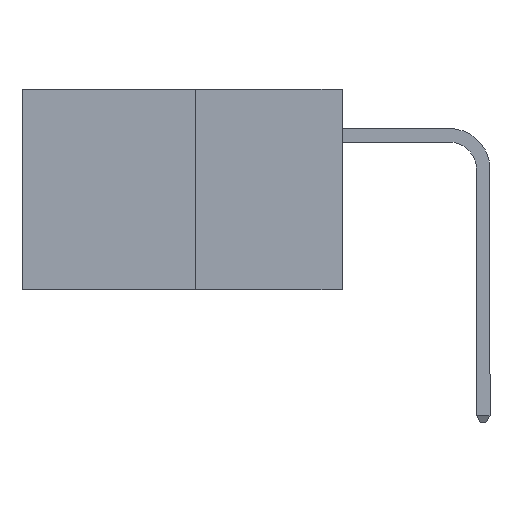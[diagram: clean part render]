
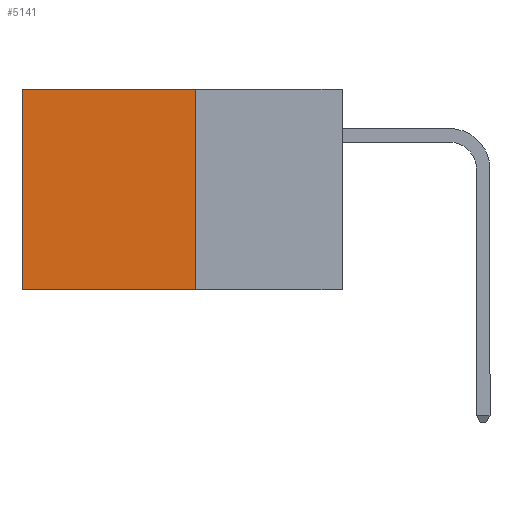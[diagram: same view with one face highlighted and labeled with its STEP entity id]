
A CAD part, left-side view. The second image highlights one B-rep face of the part: STEP entity #5141.
In plain terms, the highlighted planar face has unit normal (-1, 0, 0).
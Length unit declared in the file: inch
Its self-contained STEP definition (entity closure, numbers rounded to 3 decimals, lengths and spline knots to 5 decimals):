
#7 = LINE ( 'NONE', #8174, #3873 ) ;
#1170 = EDGE_LOOP ( 'NONE', ( #4244, #2759, #6748, #7201 ) ) ;
#1661 = VERTEX_POINT ( 'NONE', #3243 ) ;
#1672 = EDGE_CURVE ( 'NONE', #7537, #4036, #6747, .T. ) ;
#1724 = VERTEX_POINT ( 'NONE', #7793 ) ;
#2165 = LINE ( 'NONE', #4706, #3596 ) ;
#2404 = VECTOR ( 'NONE', #2428, 39.37008 ) ;
#2428 = DIRECTION ( 'NONE',  ( 0., 0., -1. ) ) ;
#2453 = EDGE_CURVE ( 'NONE', #1661, #1724, #7, .T. ) ;
#2570 = CARTESIAN_POINT ( 'NONE',  ( 0.277, 0.59, -0.37 ) ) ;
#2619 = LINE ( 'NONE', #6888, #2404 ) ;
#2759 = ORIENTED_EDGE ( 'NONE', *, *, #1672, .F. ) ;
#3243 = CARTESIAN_POINT ( 'NONE',  ( 0.277, 0.27, 0. ) ) ;
#3267 = DIRECTION ( 'NONE',  ( 0., 1., 0. ) ) ;
#3596 = VECTOR ( 'NONE', #3936, 39.37008 ) ;
#3873 = VECTOR ( 'NONE', #5328, 39.37008 ) ;
#3936 = DIRECTION ( 'NONE',  ( 0., 0., -1. ) ) ;
#4036 = VERTEX_POINT ( 'NONE', #2570 ) ;
#4162 = CARTESIAN_POINT ( 'NONE',  ( 0.277, 0.27, -0.37 ) ) ;
#4244 = ORIENTED_EDGE ( 'NONE', *, *, #9126, .T. ) ;
#4706 = CARTESIAN_POINT ( 'NONE',  ( 0.277, 0.59, -0.37 ) ) ;
#5141 = ADVANCED_FACE ( 'NONE', ( #9236 ), #7254, .F. ) ;
#5328 = DIRECTION ( 'NONE',  ( 0., 1., 0. ) ) ;
#6203 = AXIS2_PLACEMENT_3D ( 'NONE', #7246, #7221, #7155 ) ;
#6336 = CARTESIAN_POINT ( 'NONE',  ( 0.277, 0.27, -0.37 ) ) ;
#6747 = LINE ( 'NONE', #6336, #7200 ) ;
#6748 = ORIENTED_EDGE ( 'NONE', *, *, #9047, .F. ) ;
#6888 = CARTESIAN_POINT ( 'NONE',  ( 0.277, 0.27, -0.37 ) ) ;
#7155 = DIRECTION ( 'NONE',  ( 0., 0., -1. ) ) ;
#7200 = VECTOR ( 'NONE', #3267, 39.37008 ) ;
#7201 = ORIENTED_EDGE ( 'NONE', *, *, #2453, .T. ) ;
#7221 = DIRECTION ( 'NONE',  ( 1., 0., 0. ) ) ;
#7246 = CARTESIAN_POINT ( 'NONE',  ( 0.277, 0.27, -0.37 ) ) ;
#7254 = PLANE ( 'NONE',  #6203 ) ;
#7537 = VERTEX_POINT ( 'NONE', #4162 ) ;
#7793 = CARTESIAN_POINT ( 'NONE',  ( 0.277, 0.59, 0. ) ) ;
#8174 = CARTESIAN_POINT ( 'NONE',  ( 0.277, 0.27, 0. ) ) ;
#9047 = EDGE_CURVE ( 'NONE', #1661, #7537, #2619, .T. ) ;
#9126 = EDGE_CURVE ( 'NONE', #1724, #4036, #2165, .T. ) ;
#9236 = FACE_OUTER_BOUND ( 'NONE', #1170, .T. ) ;
